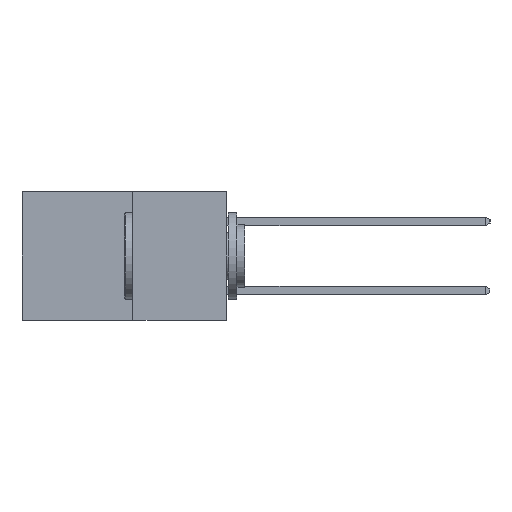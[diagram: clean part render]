
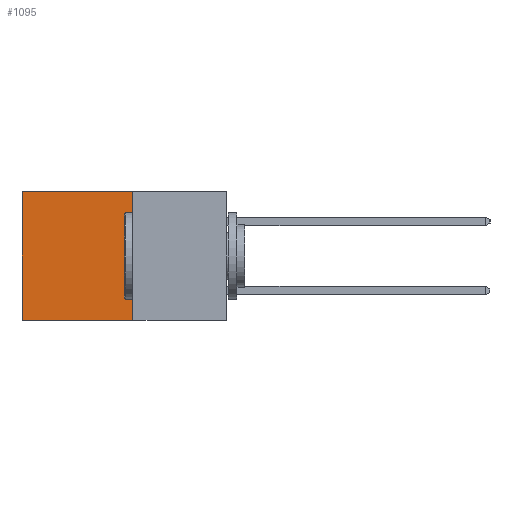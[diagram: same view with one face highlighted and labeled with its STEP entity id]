
A CAD part, left-side view. The second image highlights one B-rep face of the part: STEP entity #1095.
In plain terms, the highlighted planar face has unit normal (-1, 0, 0).
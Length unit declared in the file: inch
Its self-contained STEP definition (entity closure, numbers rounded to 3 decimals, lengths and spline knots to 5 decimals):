
#89 = EDGE_CURVE ( 'NONE', #6542, #2956, #5397, .T. ) ;
#521 = EDGE_CURVE ( 'NONE', #2622, #5309, #5236, .T. ) ;
#1095 = ADVANCED_FACE ( 'NONE', ( #7842 ), #6879, .F. ) ;
#1929 = VECTOR ( 'NONE', #3412, 39.37008 ) ;
#2022 = VECTOR ( 'NONE', #8323, 39.37008 ) ;
#2185 = CARTESIAN_POINT ( 'NONE',  ( 0.277, 0.27, -0.37 ) ) ;
#2622 = VERTEX_POINT ( 'NONE', #3112 ) ;
#2809 = CARTESIAN_POINT ( 'NONE',  ( 0.277, 0.59, 0. ) ) ;
#2856 = AXIS2_PLACEMENT_3D ( 'NONE', #6856, #3017, #7553 ) ;
#2956 = VERTEX_POINT ( 'NONE', #6629 ) ;
#3017 = DIRECTION ( 'NONE',  ( 1., 0., 0. ) ) ;
#3112 = CARTESIAN_POINT ( 'NONE',  ( 0.277, 0.27, 0. ) ) ;
#3210 = ORIENTED_EDGE ( 'NONE', *, *, #7814, .F. ) ;
#3412 = DIRECTION ( 'NONE',  ( 0., 0., -1. ) ) ;
#3495 = EDGE_LOOP ( 'NONE', ( #8343, #3210, #7743, #4757 ) ) ;
#3583 = CARTESIAN_POINT ( 'NONE',  ( 0.277, 0.27, -0.37 ) ) ;
#3703 = VECTOR ( 'NONE', #6348, 39.37008 ) ;
#3804 = CARTESIAN_POINT ( 'NONE',  ( 0.277, 0.27, 0. ) ) ;
#4021 = CARTESIAN_POINT ( 'NONE',  ( 0.277, 0.59, -0.37 ) ) ;
#4483 = VECTOR ( 'NONE', #6708, 39.37008 ) ;
#4757 = ORIENTED_EDGE ( 'NONE', *, *, #8161, .T. ) ;
#5069 = CARTESIAN_POINT ( 'NONE',  ( 0.277, 0.27, -0.37 ) ) ;
#5236 = LINE ( 'NONE', #5069, #3703 ) ;
#5309 = VERTEX_POINT ( 'NONE', #3583 ) ;
#5397 = LINE ( 'NONE', #4021, #1929 ) ;
#6348 = DIRECTION ( 'NONE',  ( 0., 0., -1. ) ) ;
#6542 = VERTEX_POINT ( 'NONE', #2809 ) ;
#6629 = CARTESIAN_POINT ( 'NONE',  ( 0.277, 0.59, -0.37 ) ) ;
#6708 = DIRECTION ( 'NONE',  ( 0., 1., 0. ) ) ;
#6856 = CARTESIAN_POINT ( 'NONE',  ( 0.277, 0.27, -0.37 ) ) ;
#6879 = PLANE ( 'NONE',  #2856 ) ;
#6988 = LINE ( 'NONE', #3804, #2022 ) ;
#7553 = DIRECTION ( 'NONE',  ( 0., 0., -1. ) ) ;
#7743 = ORIENTED_EDGE ( 'NONE', *, *, #521, .F. ) ;
#7814 = EDGE_CURVE ( 'NONE', #5309, #2956, #8119, .T. ) ;
#7842 = FACE_OUTER_BOUND ( 'NONE', #3495, .T. ) ;
#8119 = LINE ( 'NONE', #2185, #4483 ) ;
#8161 = EDGE_CURVE ( 'NONE', #2622, #6542, #6988, .T. ) ;
#8323 = DIRECTION ( 'NONE',  ( 0., 1., 0. ) ) ;
#8343 = ORIENTED_EDGE ( 'NONE', *, *, #89, .T. ) ;
